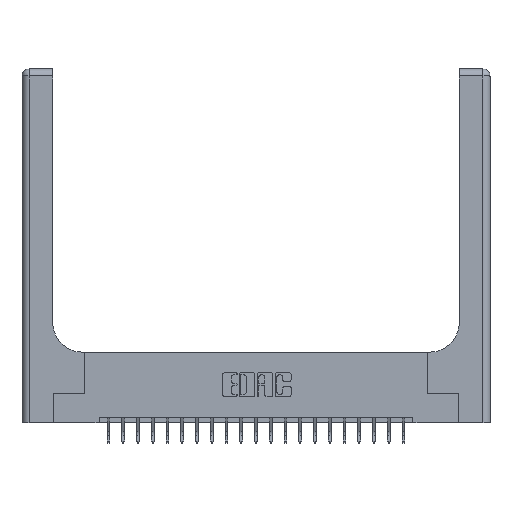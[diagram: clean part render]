
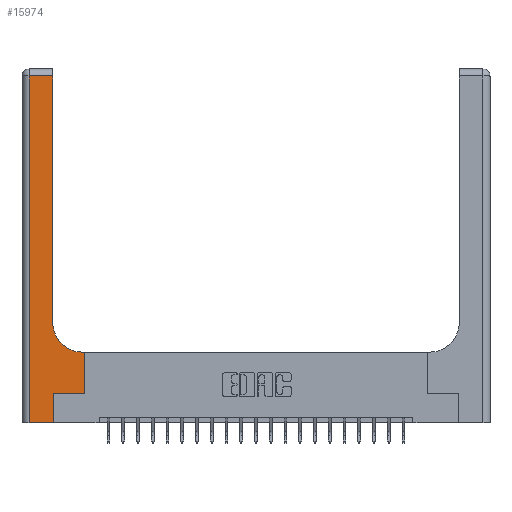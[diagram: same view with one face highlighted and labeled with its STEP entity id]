
A CAD part, top view. The second image highlights one B-rep face of the part: STEP entity #15974.
In plain terms, the highlighted planar face has unit normal (0, 0, 1).
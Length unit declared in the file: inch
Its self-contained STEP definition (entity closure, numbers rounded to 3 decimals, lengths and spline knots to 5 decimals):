
#432 = EDGE_CURVE ( 'NONE', #21135, #15876, #18707, .T. ) ;
#995 = EDGE_CURVE ( 'NONE', #21626, #16217, #15839, .T. ) ;
#1238 = CARTESIAN_POINT ( 'NONE',  ( 0., 2.94, 0.37 ) ) ;
#1646 = ORIENTED_EDGE ( 'NONE', *, *, #21609, .T. ) ;
#1690 = LINE ( 'NONE', #6696, #16525 ) ;
#1915 = CIRCLE ( 'NONE', #21107, 0.25 ) ;
#1941 = VECTOR ( 'NONE', #8567, 39.37008 ) ;
#2002 = DIRECTION ( 'NONE',  ( -1., 0., 0. ) ) ;
#2094 = VECTOR ( 'NONE', #10774, 39.37008 ) ;
#2153 = DIRECTION ( 'NONE',  ( 0., 0., -1. ) ) ;
#2881 = EDGE_CURVE ( 'NONE', #15876, #15018, #5411, .T. ) ;
#3031 = DIRECTION ( 'NONE',  ( 1., 0., 0. ) ) ;
#3080 = ORIENTED_EDGE ( 'NONE', *, *, #5880, .T. ) ;
#3144 = VECTOR ( 'NONE', #3368, 39.37008 ) ;
#3368 = DIRECTION ( 'NONE',  ( 0., 1., 0. ) ) ;
#4626 = VECTOR ( 'NONE', #2002, 39.37008 ) ;
#4793 = AXIS2_PLACEMENT_3D ( 'NONE', #15551, #2153, #19277 ) ;
#4973 = VERTEX_POINT ( 'NONE', #21688 ) ;
#5148 = CARTESIAN_POINT ( 'NONE',  ( 0.528, 0.6, 0.37 ) ) ;
#5411 = LINE ( 'NONE', #7241, #3144 ) ;
#5562 = VECTOR ( 'NONE', #16097, 39.37008 ) ;
#5673 = LINE ( 'NONE', #8851, #2094 ) ;
#5779 = CARTESIAN_POINT ( 'NONE',  ( 0.528, 0.25, 0.37 ) ) ;
#5880 = EDGE_CURVE ( 'NONE', #9011, #17720, #1690, .T. ) ;
#5907 = LINE ( 'NONE', #21635, #5562 ) ;
#6584 = DIRECTION ( 'NONE',  ( 0., 1., 0. ) ) ;
#6696 = CARTESIAN_POINT ( 'NONE',  ( 0.26, 3., 0.37 ) ) ;
#6847 = CARTESIAN_POINT ( 'NONE',  ( 0.26, 0.85, 0.37 ) ) ;
#7057 = PLANE ( 'NONE',  #4793 ) ;
#7192 = ORIENTED_EDGE ( 'NONE', *, *, #19397, .T. ) ;
#7241 = CARTESIAN_POINT ( 'NONE',  ( 0.265, 0., 0.37 ) ) ;
#8498 = VECTOR ( 'NONE', #22214, 39.37008 ) ;
#8567 = DIRECTION ( 'NONE',  ( 1., 0., 0. ) ) ;
#8851 = CARTESIAN_POINT ( 'NONE',  ( 0.06, 3., 0.37 ) ) ;
#9011 = VERTEX_POINT ( 'NONE', #6847 ) ;
#9623 = EDGE_CURVE ( 'NONE', #4973, #21135, #5673, .T. ) ;
#10108 = CARTESIAN_POINT ( 'NONE',  ( 0.265, 0.25, 0.37 ) ) ;
#10250 = CARTESIAN_POINT ( 'NONE',  ( 0.265, 0., 0.37 ) ) ;
#10332 = ORIENTED_EDGE ( 'NONE', *, *, #17963, .T. ) ;
#10774 = DIRECTION ( 'NONE',  ( 0., -1., 0. ) ) ;
#11006 = CARTESIAN_POINT ( 'NONE',  ( 0.26, 2.94, 0.37 ) ) ;
#11213 = ORIENTED_EDGE ( 'NONE', *, *, #17805, .T. ) ;
#12177 = LINE ( 'NONE', #12397, #1941 ) ;
#12397 = CARTESIAN_POINT ( 'NONE',  ( 0.265, 0.25, 0.37 ) ) ;
#12620 = FACE_OUTER_BOUND ( 'NONE', #19333, .T. ) ;
#13256 = DIRECTION ( 'NONE',  ( -1., 0., 0. ) ) ;
#13608 = CARTESIAN_POINT ( 'NONE',  ( 0.51, 0.85, 0.37 ) ) ;
#13639 = VECTOR ( 'NONE', #13256, 39.37008 ) ;
#14043 = CARTESIAN_POINT ( 'NONE',  ( 0.26, 0.6, 0.37 ) ) ;
#15018 = VERTEX_POINT ( 'NONE', #10108 ) ;
#15290 = DIRECTION ( 'NONE',  ( 0., 0., -1. ) ) ;
#15342 = ORIENTED_EDGE ( 'NONE', *, *, #9623, .T. ) ;
#15551 = CARTESIAN_POINT ( 'NONE',  ( 0., 3., 0.37 ) ) ;
#15706 = ORIENTED_EDGE ( 'NONE', *, *, #2881, .T. ) ;
#15839 = LINE ( 'NONE', #14043, #4626 ) ;
#15876 = VERTEX_POINT ( 'NONE', #10250 ) ;
#15974 = ADVANCED_FACE ( 'NONE', ( #12620 ), #7057, .F. ) ;
#16097 = DIRECTION ( 'NONE',  ( 0., 1., 0. ) ) ;
#16217 = VERTEX_POINT ( 'NONE', #16783 ) ;
#16525 = VECTOR ( 'NONE', #6584, 39.37008 ) ;
#16766 = LINE ( 'NONE', #1238, #13639 ) ;
#16783 = CARTESIAN_POINT ( 'NONE',  ( 0.51, 0.6, 0.37 ) ) ;
#17720 = VERTEX_POINT ( 'NONE', #11006 ) ;
#17805 = EDGE_CURVE ( 'NONE', #19623, #21626, #5907, .T. ) ;
#17963 = EDGE_CURVE ( 'NONE', #16217, #9011, #1915, .T. ) ;
#18233 = ORIENTED_EDGE ( 'NONE', *, *, #432, .T. ) ;
#18707 = LINE ( 'NONE', #18914, #8498 ) ;
#18914 = CARTESIAN_POINT ( 'NONE',  ( 0., 0., 0.37 ) ) ;
#19277 = DIRECTION ( 'NONE',  ( -1., 0., 0. ) ) ;
#19333 = EDGE_LOOP ( 'NONE', ( #3080, #7192, #15342, #18233, #15706, #1646, #11213, #22180, #10332 ) ) ;
#19397 = EDGE_CURVE ( 'NONE', #17720, #4973, #16766, .T. ) ;
#19623 = VERTEX_POINT ( 'NONE', #5779 ) ;
#21107 = AXIS2_PLACEMENT_3D ( 'NONE', #13608, #15290, #3031 ) ;
#21133 = CARTESIAN_POINT ( 'NONE',  ( 0.06, 0., 0.37 ) ) ;
#21135 = VERTEX_POINT ( 'NONE', #21133 ) ;
#21609 = EDGE_CURVE ( 'NONE', #15018, #19623, #12177, .T. ) ;
#21626 = VERTEX_POINT ( 'NONE', #5148 ) ;
#21635 = CARTESIAN_POINT ( 'NONE',  ( 0.528, 0.25, 0.37 ) ) ;
#21688 = CARTESIAN_POINT ( 'NONE',  ( 0.06, 2.94, 0.37 ) ) ;
#22180 = ORIENTED_EDGE ( 'NONE', *, *, #995, .T. ) ;
#22214 = DIRECTION ( 'NONE',  ( 1., 0., 0. ) ) ;
